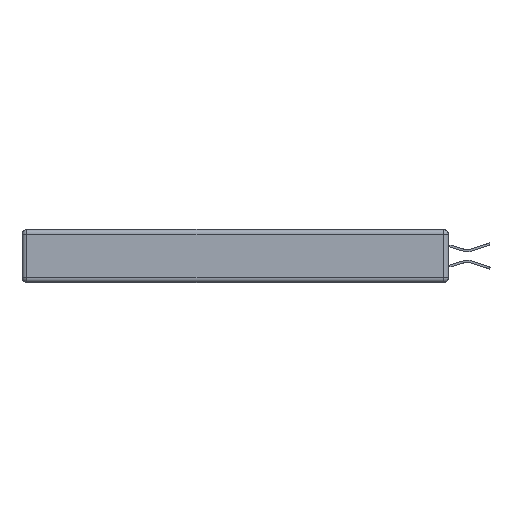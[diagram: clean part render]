
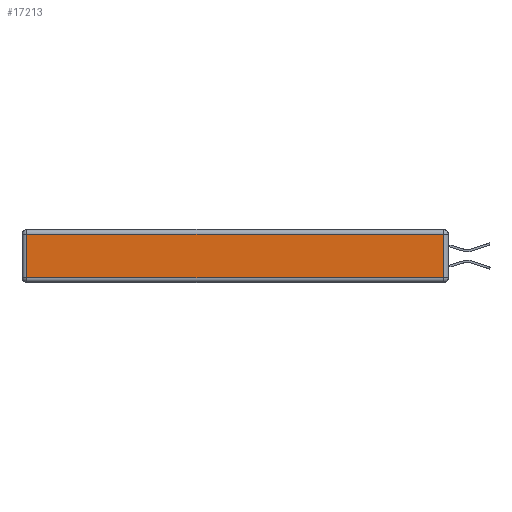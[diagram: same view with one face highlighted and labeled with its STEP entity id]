
A CAD part, left-side view. The second image highlights one B-rep face of the part: STEP entity #17213.
In plain terms, the highlighted planar face has unit normal (-1, 0, 0).
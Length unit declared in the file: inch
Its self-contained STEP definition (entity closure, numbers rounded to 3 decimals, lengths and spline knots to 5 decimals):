
#883 = AXIS2_PLACEMENT_3D ( 'NONE', #7774, #20618, #22490 ) ;
#1125 = CARTESIAN_POINT ( 'NONE',  ( 0., 0., -0.313 ) ) ;
#1540 = LINE ( 'NONE', #13156, #12746 ) ;
#3732 = LINE ( 'NONE', #9689, #17060 ) ;
#4266 = DIRECTION ( 'NONE',  ( 0., 1., 0. ) ) ;
#5054 = VERTEX_POINT ( 'NONE', #19702 ) ;
#6284 = ORIENTED_EDGE ( 'NONE', *, *, #18812, .T. ) ;
#6839 = CARTESIAN_POINT ( 'NONE',  ( 0., 2.72, -0.03 ) ) ;
#7207 = FACE_OUTER_BOUND ( 'NONE', #8655, .T. ) ;
#7774 = CARTESIAN_POINT ( 'NONE',  ( 0., 0., -0.343 ) ) ;
#8655 = EDGE_LOOP ( 'NONE', ( #6284, #20659, #20278, #9375 ) ) ;
#9375 = ORIENTED_EDGE ( 'NONE', *, *, #10506, .T. ) ;
#9689 = CARTESIAN_POINT ( 'NONE',  ( 0., 2.72, -0.343 ) ) ;
#10506 = EDGE_CURVE ( 'NONE', #17247, #14525, #3732, .T. ) ;
#10859 = CARTESIAN_POINT ( 'NONE',  ( 0., 2.72, -0.313 ) ) ;
#11806 = DIRECTION ( 'NONE',  ( 0., -1., 0. ) ) ;
#12746 = VECTOR ( 'NONE', #16768, 39.37008 ) ;
#13156 = CARTESIAN_POINT ( 'NONE',  ( 0., 0.03, -0.343 ) ) ;
#13207 = PLANE ( 'NONE',  #883 ) ;
#13584 = CARTESIAN_POINT ( 'NONE',  ( 0., 2.75, -0.03 ) ) ;
#14525 = VERTEX_POINT ( 'NONE', #10859 ) ;
#16768 = DIRECTION ( 'NONE',  ( 0., 0., 1. ) ) ;
#17060 = VECTOR ( 'NONE', #22582, 39.37008 ) ;
#17213 = ADVANCED_FACE ( 'NONE', ( #7207 ), #13207, .T. ) ;
#17247 = VERTEX_POINT ( 'NONE', #6839 ) ;
#18199 = EDGE_CURVE ( 'NONE', #5054, #17247, #20372, .T. ) ;
#18273 = VERTEX_POINT ( 'NONE', #22799 ) ;
#18812 = EDGE_CURVE ( 'NONE', #14525, #18273, #19195, .T. ) ;
#19195 = LINE ( 'NONE', #1125, #19486 ) ;
#19486 = VECTOR ( 'NONE', #11806, 39.37008 ) ;
#19702 = CARTESIAN_POINT ( 'NONE',  ( 0., 0.03, -0.03 ) ) ;
#20235 = EDGE_CURVE ( 'NONE', #18273, #5054, #1540, .T. ) ;
#20278 = ORIENTED_EDGE ( 'NONE', *, *, #18199, .T. ) ;
#20372 = LINE ( 'NONE', #13584, #22711 ) ;
#20618 = DIRECTION ( 'NONE',  ( -1., 0., 0. ) ) ;
#20659 = ORIENTED_EDGE ( 'NONE', *, *, #20235, .T. ) ;
#22490 = DIRECTION ( 'NONE',  ( 0., 0., 1. ) ) ;
#22582 = DIRECTION ( 'NONE',  ( 0., 0., -1. ) ) ;
#22711 = VECTOR ( 'NONE', #4266, 39.37008 ) ;
#22799 = CARTESIAN_POINT ( 'NONE',  ( 0., 0.03, -0.313 ) ) ;
